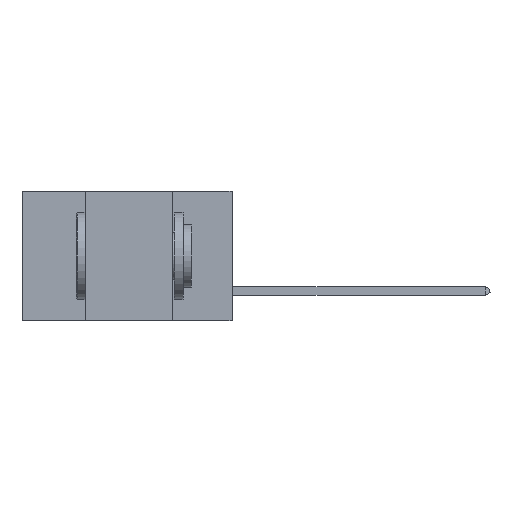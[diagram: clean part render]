
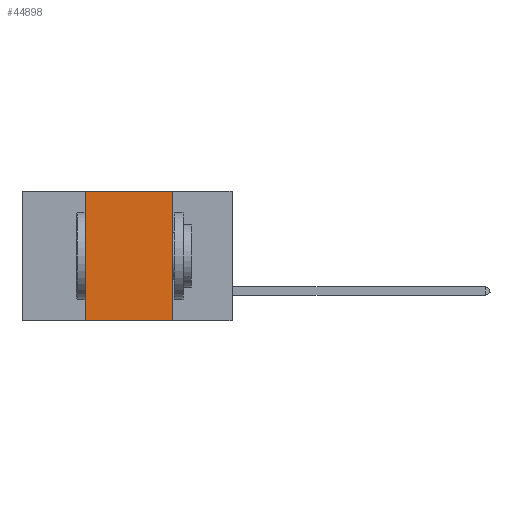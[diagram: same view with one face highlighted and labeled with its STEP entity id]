
A CAD part, left-side view. The second image highlights one B-rep face of the part: STEP entity #44898.
In plain terms, the highlighted planar face has unit normal (-1, 0, 0).
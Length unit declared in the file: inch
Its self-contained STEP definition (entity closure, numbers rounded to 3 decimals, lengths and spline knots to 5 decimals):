
#118 = CARTESIAN_POINT ( 'NONE',  ( 0., 0.17, 0. ) ) ;
#303 = CARTESIAN_POINT ( 'NONE',  ( 0., 0.42, 0. ) ) ;
#496 = VERTEX_POINT ( 'NONE', #11791 ) ;
#972 = FACE_OUTER_BOUND ( 'NONE', #37930, .T. ) ;
#1074 = VERTEX_POINT ( 'NONE', #28755 ) ;
#2556 = ORIENTED_EDGE ( 'NONE', *, *, #18664, .F. ) ;
#3775 = CARTESIAN_POINT ( 'NONE',  ( 0., 0.6, 0. ) ) ;
#3908 = ORIENTED_EDGE ( 'NONE', *, *, #30598, .F. ) ;
#5613 = ORIENTED_EDGE ( 'NONE', *, *, #44712, .F. ) ;
#6034 = VECTOR ( 'NONE', #19198, 39.37008 ) ;
#7177 = VERTEX_POINT ( 'NONE', #46584 ) ;
#7563 = LINE ( 'NONE', #36774, #32495 ) ;
#7780 = LINE ( 'NONE', #3775, #6034 ) ;
#8652 = DIRECTION ( 'NONE',  ( 1., 0., 0. ) ) ;
#11721 = ORIENTED_EDGE ( 'NONE', *, *, #40118, .T. ) ;
#11791 = CARTESIAN_POINT ( 'NONE',  ( 0., 0.42, -0.37 ) ) ;
#12789 = CARTESIAN_POINT ( 'NONE',  ( 0., 0.6, 0. ) ) ;
#14030 = DIRECTION ( 'NONE',  ( 0., -1., 0. ) ) ;
#15169 = LINE ( 'NONE', #118, #47851 ) ;
#18664 = EDGE_CURVE ( 'NONE', #7177, #30652, #7780, .T. ) ;
#19198 = DIRECTION ( 'NONE',  ( 0., -1., 0. ) ) ;
#21763 = LINE ( 'NONE', #303, #39627 ) ;
#23524 = CARTESIAN_POINT ( 'NONE',  ( 0., 0.17, 0. ) ) ;
#28755 = CARTESIAN_POINT ( 'NONE',  ( 0., 0.17, -0.37 ) ) ;
#30598 = EDGE_CURVE ( 'NONE', #30652, #1074, #15169, .T. ) ;
#30652 = VERTEX_POINT ( 'NONE', #23524 ) ;
#31997 = PLANE ( 'NONE',  #42767 ) ;
#32495 = VECTOR ( 'NONE', #14030, 39.37008 ) ;
#34331 = DIRECTION ( 'NONE',  ( 0., 0., -1. ) ) ;
#35014 = DIRECTION ( 'NONE',  ( 0., 0., -1. ) ) ;
#36774 = CARTESIAN_POINT ( 'NONE',  ( 0., 0.6, -0.37 ) ) ;
#37930 = EDGE_LOOP ( 'NONE', ( #3908, #2556, #5613, #11721 ) ) ;
#39627 = VECTOR ( 'NONE', #41826, 39.37008 ) ;
#40118 = EDGE_CURVE ( 'NONE', #496, #1074, #7563, .T. ) ;
#41826 = DIRECTION ( 'NONE',  ( 0., 0., 1. ) ) ;
#42767 = AXIS2_PLACEMENT_3D ( 'NONE', #12789, #8652, #35014 ) ;
#44712 = EDGE_CURVE ( 'NONE', #496, #7177, #21763, .T. ) ;
#44898 = ADVANCED_FACE ( 'NONE', ( #972 ), #31997, .F. ) ;
#46584 = CARTESIAN_POINT ( 'NONE',  ( 0., 0.42, 0. ) ) ;
#47851 = VECTOR ( 'NONE', #34331, 39.37008 ) ;
